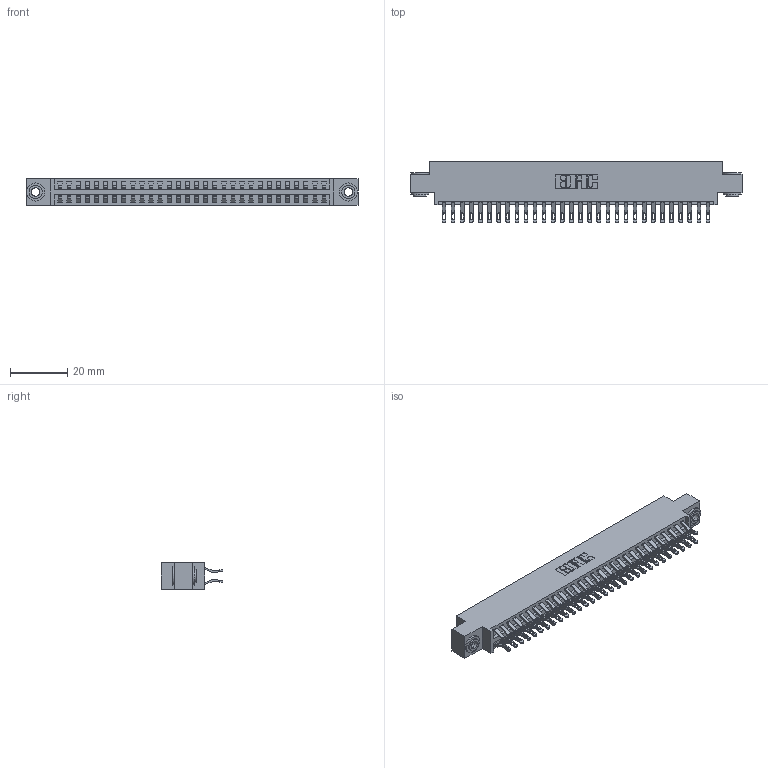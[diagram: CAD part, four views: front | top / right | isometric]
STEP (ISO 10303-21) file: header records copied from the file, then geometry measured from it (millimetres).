
FILE_DESCRIPTION (( 'STEP AP203' ), '1' );
FILE_NAME ('346-060-555-803.STEP', '2022-05-21T11:52:30', ( '' ), ( '' ), 'SwSTEP 2.0', 'SolidWorks 2020', '' );
FILE_SCHEMA (( 'CONFIG_CONTROL_DESIGN' ));
Length unit declared in the file: inch
Products named in the file (4): 346-060-555-803; 345-292-001_555 Tail; 346 Part_0.170 Offset - 0.156 Dia-TH; 345-250-002_345-250-002-102
Assembly tree (63 placements, depth 2):
  346-060-555-803
    346 Part_0.170 Offset - 0.156 Dia-TH
    345-292-001_555 Tail  x60
    345-250-002_345-250-002-102  x2
Bounding box: 115.82 x 21.46 x 9.4 mm (x, y, z)
Volume: 11221.8 mm3; surface area: 16285.2 mm2
Topology: 63 solids, 63 shells, 3658 faces, 11433 edges, 7618 vertices
Faces by surface type: plane 2084, cylinder 1566, cone 8
Entity records: 22718 total; most frequent: CARTESIAN_POINT 3779, ORIENTED_EDGE 3674, DIRECTION 3379, EDGE_CURVE 1837, LINE 1541, VECTOR 1541, VERTEX_POINT 1222, AXIS2_PLACEMENT_3D 919
